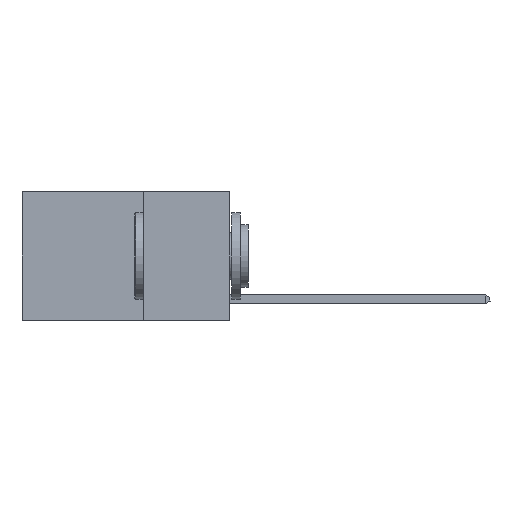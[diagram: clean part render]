
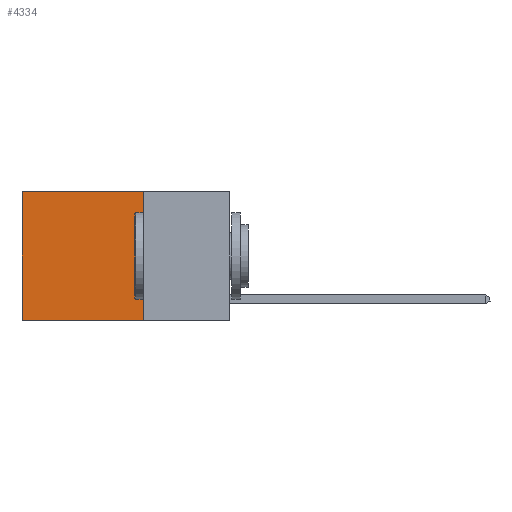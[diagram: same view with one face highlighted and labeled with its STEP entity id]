
A CAD part, left-side view. The second image highlights one B-rep face of the part: STEP entity #4334.
In plain terms, the highlighted planar face has unit normal (-1, 0, 0).
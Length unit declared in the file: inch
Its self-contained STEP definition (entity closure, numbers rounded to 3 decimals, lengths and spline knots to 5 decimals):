
#50 = CARTESIAN_POINT ( 'NONE',  ( 0.2625, 0.25, 0. ) ) ;
#286 = ORIENTED_EDGE ( 'NONE', *, *, #11275, .F. ) ;
#318 = VERTEX_POINT ( 'NONE', #13035 ) ;
#408 = VERTEX_POINT ( 'NONE', #50 ) ;
#422 = DIRECTION ( 'NONE',  ( 1., 0., 0. ) ) ;
#814 = VECTOR ( 'NONE', #4401, 39.37008 ) ;
#977 = DIRECTION ( 'NONE',  ( 0., 1., 0. ) ) ;
#1081 = ORIENTED_EDGE ( 'NONE', *, *, #8530, .F. ) ;
#1453 = CARTESIAN_POINT ( 'NONE',  ( 0.2625, 0.25, 0. ) ) ;
#1514 = DIRECTION ( 'NONE',  ( 0., 0., -1. ) ) ;
#1830 = VECTOR ( 'NONE', #977, 39.37008 ) ;
#2010 = ORIENTED_EDGE ( 'NONE', *, *, #5608, .T. ) ;
#2235 = CARTESIAN_POINT ( 'NONE',  ( 0.2625, 0.25, -0.37 ) ) ;
#3895 = EDGE_CURVE ( 'NONE', #10918, #318, #7615, .T. ) ;
#3952 = VECTOR ( 'NONE', #4557, 39.37008 ) ;
#4165 = VECTOR ( 'NONE', #7683, 39.37008 ) ;
#4203 = EDGE_LOOP ( 'NONE', ( #7192, #286, #1081, #2010 ) ) ;
#4334 = ADVANCED_FACE ( 'NONE', ( #7595 ), #6624, .F. ) ;
#4401 = DIRECTION ( 'NONE',  ( 0., 0., -1. ) ) ;
#4557 = DIRECTION ( 'NONE',  ( 0., 1., 0. ) ) ;
#4687 = LINE ( 'NONE', #5545, #3952 ) ;
#4828 = AXIS2_PLACEMENT_3D ( 'NONE', #1453, #422, #1514 ) ;
#5446 = CARTESIAN_POINT ( 'NONE',  ( 0.2625, 0.6, 0. ) ) ;
#5545 = CARTESIAN_POINT ( 'NONE',  ( 0.2625, 0.25, -0.37 ) ) ;
#5608 = EDGE_CURVE ( 'NONE', #408, #10918, #9266, .T. ) ;
#6624 = PLANE ( 'NONE',  #4828 ) ;
#7192 = ORIENTED_EDGE ( 'NONE', *, *, #3895, .T. ) ;
#7595 = FACE_OUTER_BOUND ( 'NONE', #4203, .T. ) ;
#7615 = LINE ( 'NONE', #5446, #4165 ) ;
#7683 = DIRECTION ( 'NONE',  ( 0., 0., -1. ) ) ;
#8490 = CARTESIAN_POINT ( 'NONE',  ( 0.2625, 0.25, 0. ) ) ;
#8530 = EDGE_CURVE ( 'NONE', #408, #11066, #9484, .T. ) ;
#9266 = LINE ( 'NONE', #8490, #1830 ) ;
#9484 = LINE ( 'NONE', #9612, #814 ) ;
#9612 = CARTESIAN_POINT ( 'NONE',  ( 0.2625, 0.25, 0. ) ) ;
#10918 = VERTEX_POINT ( 'NONE', #12201 ) ;
#11066 = VERTEX_POINT ( 'NONE', #2235 ) ;
#11275 = EDGE_CURVE ( 'NONE', #11066, #318, #4687, .T. ) ;
#12201 = CARTESIAN_POINT ( 'NONE',  ( 0.2625, 0.6, 0. ) ) ;
#13035 = CARTESIAN_POINT ( 'NONE',  ( 0.2625, 0.6, -0.37 ) ) ;
